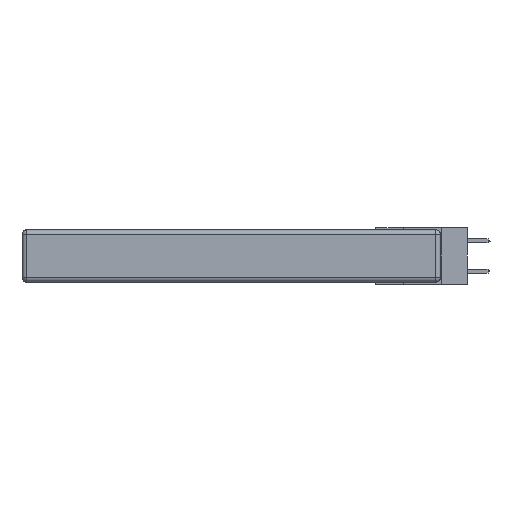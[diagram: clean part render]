
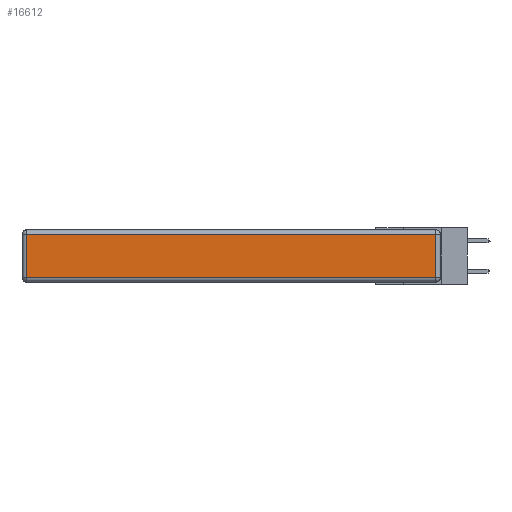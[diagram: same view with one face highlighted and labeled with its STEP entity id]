
A CAD part, left-side view. The second image highlights one B-rep face of the part: STEP entity #16612.
In plain terms, the highlighted planar face has unit normal (-1, 0, 0).
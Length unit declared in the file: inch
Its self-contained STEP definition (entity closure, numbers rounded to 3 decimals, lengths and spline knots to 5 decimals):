
#585 = CARTESIAN_POINT ( 'NONE',  ( 0., 2.72, -0.03 ) ) ;
#809 = LINE ( 'NONE', #18257, #28250 ) ;
#1292 = EDGE_CURVE ( 'NONE', #7847, #7031, #5700, .T. ) ;
#1698 = CARTESIAN_POINT ( 'NONE',  ( 0., 0., -0.343 ) ) ;
#2100 = CARTESIAN_POINT ( 'NONE',  ( 0., 2.72, -0.343 ) ) ;
#3403 = DIRECTION ( 'NONE',  ( 0., 1., 0. ) ) ;
#3814 = ORIENTED_EDGE ( 'NONE', *, *, #1292, .T. ) ;
#4413 = EDGE_CURVE ( 'NONE', #7031, #13561, #27835, .T. ) ;
#5700 = LINE ( 'NONE', #23105, #13727 ) ;
#7031 = VERTEX_POINT ( 'NONE', #7286 ) ;
#7286 = CARTESIAN_POINT ( 'NONE',  ( 0., 0.03, -0.03 ) ) ;
#7847 = VERTEX_POINT ( 'NONE', #22206 ) ;
#8714 = LINE ( 'NONE', #2100, #13842 ) ;
#10057 = ORIENTED_EDGE ( 'NONE', *, *, #22425, .T. ) ;
#13030 = VERTEX_POINT ( 'NONE', #20185 ) ;
#13453 = DIRECTION ( 'NONE',  ( -1., 0., 0. ) ) ;
#13561 = VERTEX_POINT ( 'NONE', #585 ) ;
#13727 = VECTOR ( 'NONE', #13813, 39.37008 ) ;
#13813 = DIRECTION ( 'NONE',  ( 0., 0., 1. ) ) ;
#13842 = VECTOR ( 'NONE', #22888, 39.37008 ) ;
#15900 = ORIENTED_EDGE ( 'NONE', *, *, #26245, .T. ) ;
#16612 = ADVANCED_FACE ( 'NONE', ( #16691 ), #18155, .T. ) ;
#16691 = FACE_OUTER_BOUND ( 'NONE', #19889, .T. ) ;
#17627 = CARTESIAN_POINT ( 'NONE',  ( 0., 2.75, -0.03 ) ) ;
#18155 = PLANE ( 'NONE',  #28900 ) ;
#18257 = CARTESIAN_POINT ( 'NONE',  ( 0., 0., -0.313 ) ) ;
#19194 = ORIENTED_EDGE ( 'NONE', *, *, #4413, .T. ) ;
#19889 = EDGE_LOOP ( 'NONE', ( #10057, #3814, #19194, #15900 ) ) ;
#20185 = CARTESIAN_POINT ( 'NONE',  ( 0., 2.72, -0.313 ) ) ;
#22206 = CARTESIAN_POINT ( 'NONE',  ( 0., 0.03, -0.313 ) ) ;
#22425 = EDGE_CURVE ( 'NONE', #13030, #7847, #809, .T. ) ;
#22888 = DIRECTION ( 'NONE',  ( 0., 0., -1. ) ) ;
#23105 = CARTESIAN_POINT ( 'NONE',  ( 0., 0.03, -0.343 ) ) ;
#25037 = DIRECTION ( 'NONE',  ( 0., -1., 0. ) ) ;
#26245 = EDGE_CURVE ( 'NONE', #13561, #13030, #8714, .T. ) ;
#27183 = DIRECTION ( 'NONE',  ( 0., 0., 1. ) ) ;
#27835 = LINE ( 'NONE', #17627, #29360 ) ;
#28250 = VECTOR ( 'NONE', #25037, 39.37008 ) ;
#28900 = AXIS2_PLACEMENT_3D ( 'NONE', #1698, #13453, #27183 ) ;
#29360 = VECTOR ( 'NONE', #3403, 39.37008 ) ;
